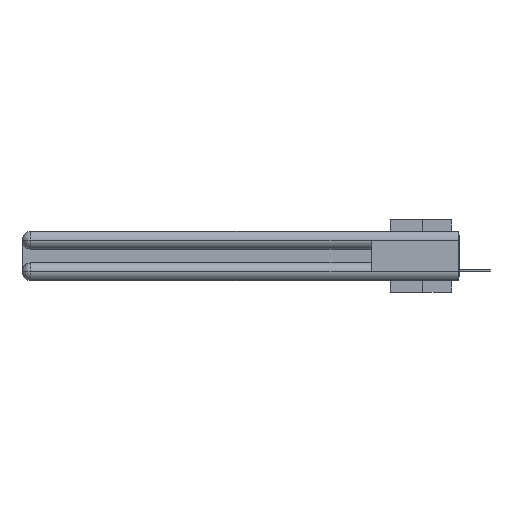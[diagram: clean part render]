
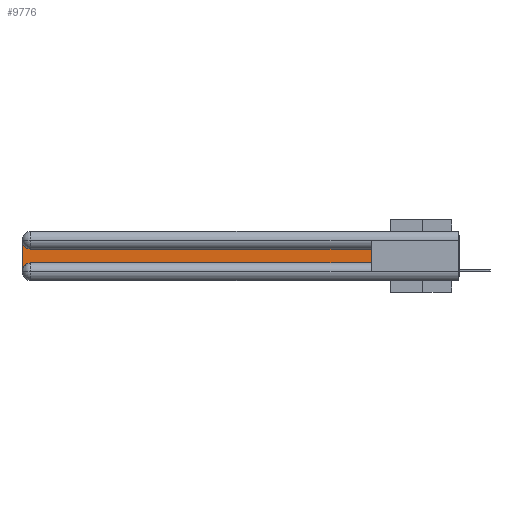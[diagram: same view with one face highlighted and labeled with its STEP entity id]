
A CAD part, left-side view. The second image highlights one B-rep face of the part: STEP entity #9776.
In plain terms, the highlighted planar face has unit normal (-1, 0, 0).
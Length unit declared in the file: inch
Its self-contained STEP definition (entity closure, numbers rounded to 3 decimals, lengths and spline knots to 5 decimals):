
#300 = LINE ( 'NONE', #28088, #17389 ) ;
#672 = FACE_OUTER_BOUND ( 'NONE', #30345, .T. ) ;
#1220 = ORIENTED_EDGE ( 'NONE', *, *, #4953, .T. ) ;
#1353 = VERTEX_POINT ( 'NONE', #29864 ) ;
#1838 = CARTESIAN_POINT ( 'NONE',  ( 0.075, 2.94, -0.0625 ) ) ;
#1953 = AXIS2_PLACEMENT_3D ( 'NONE', #9874, #14647, #22841 ) ;
#4021 = CARTESIAN_POINT ( 'NONE',  ( 0.075, 3., -0.2775 ) ) ;
#4942 = CARTESIAN_POINT ( 'NONE',  ( 0.075, 2.94, -0.1225 ) ) ;
#4953 = EDGE_CURVE ( 'NONE', #12459, #15998, #16385, .T. ) ;
#5502 = VERTEX_POINT ( 'NONE', #17821 ) ;
#5831 = VERTEX_POINT ( 'NONE', #4021 ) ;
#5977 = EDGE_CURVE ( 'NONE', #5502, #5831, #24446, .T. ) ;
#6136 = CIRCLE ( 'NONE', #30988, 0.06 ) ;
#6290 = EDGE_CURVE ( 'NONE', #5831, #7769, #6136, .T. ) ;
#7130 = CARTESIAN_POINT ( 'NONE',  ( 0.075, 0.6, -0.1225 ) ) ;
#7769 = VERTEX_POINT ( 'NONE', #25269 ) ;
#8479 = DIRECTION ( 'NONE',  ( 0., -1., 0. ) ) ;
#9563 = DIRECTION ( 'NONE',  ( 0., 0., -1. ) ) ;
#9776 = ADVANCED_FACE ( 'NONE', ( #672 ), #30164, .F. ) ;
#9874 = CARTESIAN_POINT ( 'NONE',  ( 0.075, 3., -0.1225 ) ) ;
#12373 = CARTESIAN_POINT ( 'NONE',  ( 0.075, 3., -0.2175 ) ) ;
#12459 = VERTEX_POINT ( 'NONE', #7130 ) ;
#12732 = CARTESIAN_POINT ( 'NONE',  ( 0.075, 0.6, -0.1225 ) ) ;
#12948 = EDGE_CURVE ( 'NONE', #1353, #12459, #300, .T. ) ;
#13186 = DIRECTION ( 'NONE',  ( 0., 0., 1. ) ) ;
#13343 = CARTESIAN_POINT ( 'NONE',  ( 0.075, 0.6, -0.2175 ) ) ;
#13568 = ORIENTED_EDGE ( 'NONE', *, *, #12948, .T. ) ;
#14647 = DIRECTION ( 'NONE',  ( 1., 0., 0. ) ) ;
#15185 = EDGE_CURVE ( 'NONE', #7769, #1353, #25733, .T. ) ;
#15852 = ORIENTED_EDGE ( 'NONE', *, *, #17692, .T. ) ;
#15998 = VERTEX_POINT ( 'NONE', #4942 ) ;
#16385 = LINE ( 'NONE', #12732, #20044 ) ;
#16737 = VECTOR ( 'NONE', #18960, 39.37008 ) ;
#17389 = VECTOR ( 'NONE', #13186, 39.37008 ) ;
#17497 = DIRECTION ( 'NONE',  ( 0., 0., -1. ) ) ;
#17692 = EDGE_CURVE ( 'NONE', #15998, #5502, #27323, .T. ) ;
#17821 = CARTESIAN_POINT ( 'NONE',  ( 0.075, 3., -0.0625 ) ) ;
#17870 = DIRECTION ( 'NONE',  ( 0., 1., 0. ) ) ;
#18960 = DIRECTION ( 'NONE',  ( 0., 0., -1. ) ) ;
#19766 = DIRECTION ( 'NONE',  ( 1., 0., 0. ) ) ;
#20044 = VECTOR ( 'NONE', #17870, 39.37008 ) ;
#22507 = CARTESIAN_POINT ( 'NONE',  ( 0.075, 2.94, -0.2775 ) ) ;
#22671 = ORIENTED_EDGE ( 'NONE', *, *, #6290, .T. ) ;
#22841 = DIRECTION ( 'NONE',  ( 0., 0., -1. ) ) ;
#24446 = LINE ( 'NONE', #12373, #16737 ) ;
#25159 = AXIS2_PLACEMENT_3D ( 'NONE', #1838, #32636, #17497 ) ;
#25269 = CARTESIAN_POINT ( 'NONE',  ( 0.075, 2.94, -0.2175 ) ) ;
#25497 = ORIENTED_EDGE ( 'NONE', *, *, #15185, .T. ) ;
#25733 = LINE ( 'NONE', #13343, #26537 ) ;
#26506 = ORIENTED_EDGE ( 'NONE', *, *, #5977, .T. ) ;
#26537 = VECTOR ( 'NONE', #8479, 39.37008 ) ;
#27323 = CIRCLE ( 'NONE', #25159, 0.06 ) ;
#28088 = CARTESIAN_POINT ( 'NONE',  ( 0.075, 0.6, -0.2175 ) ) ;
#29864 = CARTESIAN_POINT ( 'NONE',  ( 0.075, 0.6, -0.2175 ) ) ;
#30164 = PLANE ( 'NONE',  #1953 ) ;
#30345 = EDGE_LOOP ( 'NONE', ( #1220, #15852, #26506, #22671, #25497, #13568 ) ) ;
#30988 = AXIS2_PLACEMENT_3D ( 'NONE', #22507, #19766, #9563 ) ;
#32636 = DIRECTION ( 'NONE',  ( 1., 0., 0. ) ) ;
